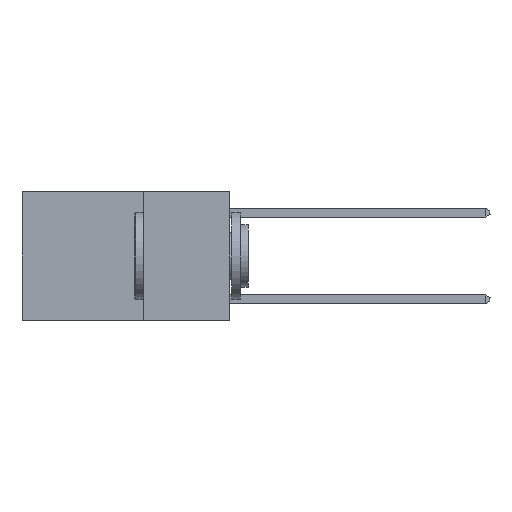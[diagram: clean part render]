
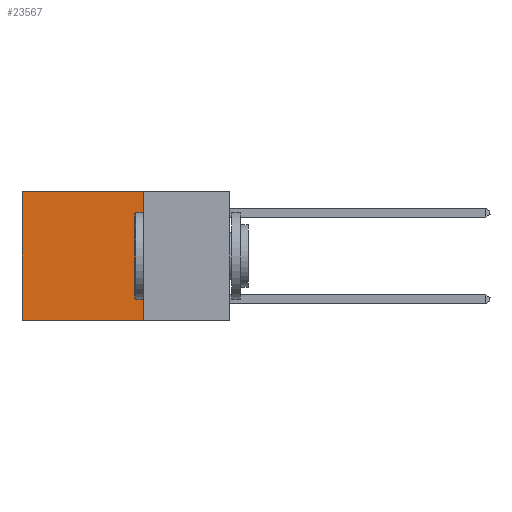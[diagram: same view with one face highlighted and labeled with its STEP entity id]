
A CAD part, left-side view. The second image highlights one B-rep face of the part: STEP entity #23567.
In plain terms, the highlighted planar face has unit normal (-1, 0, 0).
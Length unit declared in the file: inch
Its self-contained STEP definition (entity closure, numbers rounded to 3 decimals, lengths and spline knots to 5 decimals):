
#1089 = EDGE_CURVE ( 'NONE', #2562, #5010, #11994, .T. ) ;
#1446 = DIRECTION ( 'NONE',  ( 1., 0., 0. ) ) ;
#2290 = CARTESIAN_POINT ( 'NONE',  ( 0.2625, 0.25, 0. ) ) ;
#2562 = VERTEX_POINT ( 'NONE', #11786 ) ;
#2869 = ORIENTED_EDGE ( 'NONE', *, *, #13915, .F. ) ;
#4573 = VECTOR ( 'NONE', #20908, 39.37008 ) ;
#5010 = VERTEX_POINT ( 'NONE', #16032 ) ;
#5078 = DIRECTION ( 'NONE',  ( 0., 0., -1. ) ) ;
#5214 = VERTEX_POINT ( 'NONE', #2290 ) ;
#5435 = LINE ( 'NONE', #20337, #4573 ) ;
#5504 = PLANE ( 'NONE',  #19665 ) ;
#6186 = CARTESIAN_POINT ( 'NONE',  ( 0.2625, 0.6, 0. ) ) ;
#7225 = EDGE_CURVE ( 'NONE', #5214, #2562, #5435, .T. ) ;
#7347 = FACE_OUTER_BOUND ( 'NONE', #11892, .T. ) ;
#8581 = EDGE_CURVE ( 'NONE', #5214, #12428, #16440, .T. ) ;
#9110 = ORIENTED_EDGE ( 'NONE', *, *, #1089, .T. ) ;
#11786 = CARTESIAN_POINT ( 'NONE',  ( 0.2625, 0.6, 0. ) ) ;
#11892 = EDGE_LOOP ( 'NONE', ( #9110, #2869, #20924, #22375 ) ) ;
#11994 = LINE ( 'NONE', #6186, #15893 ) ;
#12428 = VERTEX_POINT ( 'NONE', #16241 ) ;
#13725 = DIRECTION ( 'NONE',  ( 0., 0., -1. ) ) ;
#13915 = EDGE_CURVE ( 'NONE', #12428, #5010, #16724, .T. ) ;
#15893 = VECTOR ( 'NONE', #13725, 39.37008 ) ;
#16032 = CARTESIAN_POINT ( 'NONE',  ( 0.2625, 0.6, -0.37 ) ) ;
#16241 = CARTESIAN_POINT ( 'NONE',  ( 0.2625, 0.25, -0.37 ) ) ;
#16316 = CARTESIAN_POINT ( 'NONE',  ( 0.2625, 0.25, 0. ) ) ;
#16440 = LINE ( 'NONE', #16316, #17529 ) ;
#16509 = DIRECTION ( 'NONE',  ( 0., 0., -1. ) ) ;
#16724 = LINE ( 'NONE', #24239, #20764 ) ;
#17529 = VECTOR ( 'NONE', #5078, 39.37008 ) ;
#18451 = CARTESIAN_POINT ( 'NONE',  ( 0.2625, 0.25, 0. ) ) ;
#18783 = DIRECTION ( 'NONE',  ( 0., 1., 0. ) ) ;
#19665 = AXIS2_PLACEMENT_3D ( 'NONE', #18451, #1446, #16509 ) ;
#20337 = CARTESIAN_POINT ( 'NONE',  ( 0.2625, 0.25, 0. ) ) ;
#20764 = VECTOR ( 'NONE', #18783, 39.37008 ) ;
#20908 = DIRECTION ( 'NONE',  ( 0., 1., 0. ) ) ;
#20924 = ORIENTED_EDGE ( 'NONE', *, *, #8581, .F. ) ;
#22375 = ORIENTED_EDGE ( 'NONE', *, *, #7225, .T. ) ;
#23567 = ADVANCED_FACE ( 'NONE', ( #7347 ), #5504, .F. ) ;
#24239 = CARTESIAN_POINT ( 'NONE',  ( 0.2625, 0.25, -0.37 ) ) ;
